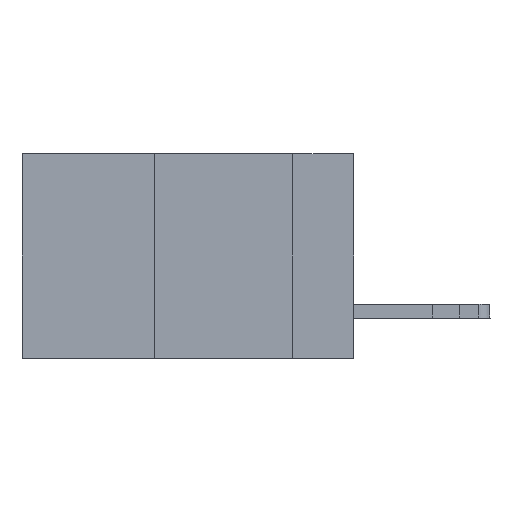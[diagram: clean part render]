
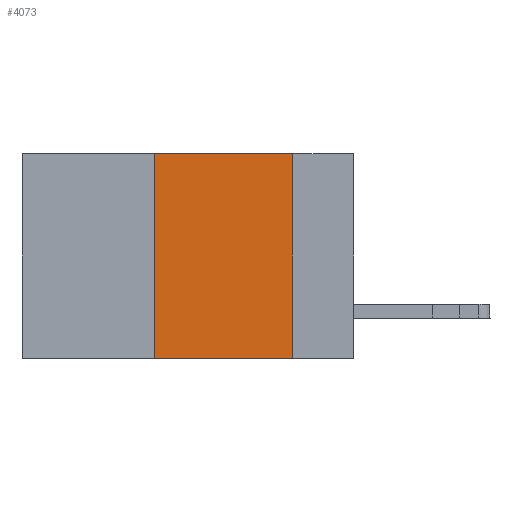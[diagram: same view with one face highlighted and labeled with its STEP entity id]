
A CAD part, left-side view. The second image highlights one B-rep face of the part: STEP entity #4073.
In plain terms, the highlighted planar face has unit normal (-1, 0, 0).
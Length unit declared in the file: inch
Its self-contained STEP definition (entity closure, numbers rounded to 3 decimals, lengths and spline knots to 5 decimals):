
#135 = VECTOR ( 'NONE', #1340, 39.37008 ) ;
#410 = VERTEX_POINT ( 'NONE', #7700 ) ;
#444 = ORIENTED_EDGE ( 'NONE', *, *, #26523, .F. ) ;
#459 = VECTOR ( 'NONE', #25932, 39.37008 ) ;
#1340 = DIRECTION ( 'NONE',  ( 0., -1., 0. ) ) ;
#2067 = CARTESIAN_POINT ( 'NONE',  ( 0., 0.6, 0. ) ) ;
#2568 = DIRECTION ( 'NONE',  ( 1., 0., 0. ) ) ;
#4073 = ADVANCED_FACE ( 'NONE', ( #22009 ), #26550, .F. ) ;
#4559 = ORIENTED_EDGE ( 'NONE', *, *, #6667, .T. ) ;
#4602 = LINE ( 'NONE', #2067, #459 ) ;
#6126 = CARTESIAN_POINT ( 'NONE',  ( 0., 0.36, 0. ) ) ;
#6444 = CARTESIAN_POINT ( 'NONE',  ( 0., 0.11, 0. ) ) ;
#6667 = EDGE_CURVE ( 'NONE', #21114, #410, #18574, .T. ) ;
#6923 = EDGE_LOOP ( 'NONE', ( #15864, #444, #13255, #4559 ) ) ;
#7408 = DIRECTION ( 'NONE',  ( 0., 0., 1. ) ) ;
#7700 = CARTESIAN_POINT ( 'NONE',  ( 0., 0.11, -0.37 ) ) ;
#8538 = CARTESIAN_POINT ( 'NONE',  ( 0., 0.6, -0.37 ) ) ;
#10349 = VERTEX_POINT ( 'NONE', #6444 ) ;
#10568 = LINE ( 'NONE', #14559, #22519 ) ;
#12248 = DIRECTION ( 'NONE',  ( 0., 0., -1. ) ) ;
#13255 = ORIENTED_EDGE ( 'NONE', *, *, #13891, .F. ) ;
#13891 = EDGE_CURVE ( 'NONE', #21114, #14879, #10568, .T. ) ;
#13991 = LINE ( 'NONE', #18942, #25901 ) ;
#14559 = CARTESIAN_POINT ( 'NONE',  ( 0., 0.36, 0. ) ) ;
#14879 = VERTEX_POINT ( 'NONE', #6126 ) ;
#15231 = CARTESIAN_POINT ( 'NONE',  ( 0., 0.36, -0.37 ) ) ;
#15864 = ORIENTED_EDGE ( 'NONE', *, *, #20495, .F. ) ;
#18574 = LINE ( 'NONE', #8538, #135 ) ;
#18942 = CARTESIAN_POINT ( 'NONE',  ( 0., 0.11, 0. ) ) ;
#20495 = EDGE_CURVE ( 'NONE', #10349, #410, #13991, .T. ) ;
#21114 = VERTEX_POINT ( 'NONE', #15231 ) ;
#21260 = AXIS2_PLACEMENT_3D ( 'NONE', #24155, #2568, #12248 ) ;
#22009 = FACE_OUTER_BOUND ( 'NONE', #6923, .T. ) ;
#22519 = VECTOR ( 'NONE', #7408, 39.37008 ) ;
#23702 = DIRECTION ( 'NONE',  ( 0., 0., -1. ) ) ;
#24155 = CARTESIAN_POINT ( 'NONE',  ( 0., 0.6, 0. ) ) ;
#25901 = VECTOR ( 'NONE', #23702, 39.37008 ) ;
#25932 = DIRECTION ( 'NONE',  ( 0., -1., 0. ) ) ;
#26523 = EDGE_CURVE ( 'NONE', #14879, #10349, #4602, .T. ) ;
#26550 = PLANE ( 'NONE',  #21260 ) ;
